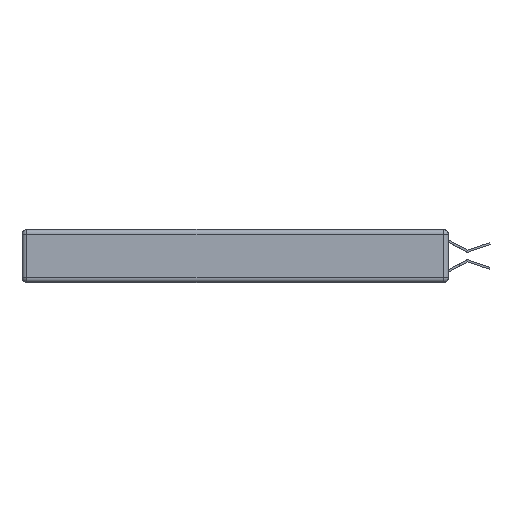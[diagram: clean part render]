
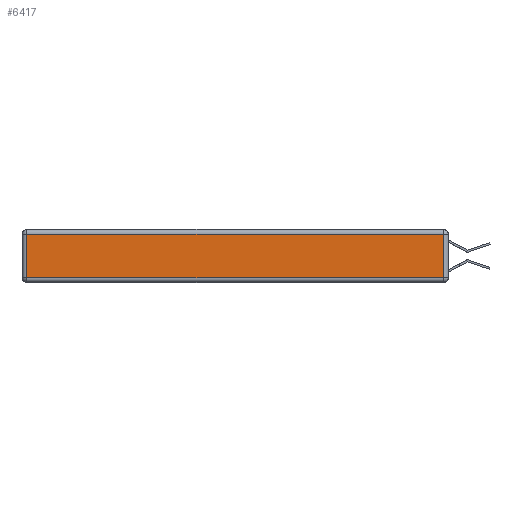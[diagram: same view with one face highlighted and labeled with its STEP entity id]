
A CAD part, left-side view. The second image highlights one B-rep face of the part: STEP entity #6417.
In plain terms, the highlighted planar face has unit normal (-1, 0, 0).
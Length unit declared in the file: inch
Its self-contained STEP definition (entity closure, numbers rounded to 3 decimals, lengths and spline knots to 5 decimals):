
#56 = VERTEX_POINT ( 'NONE', #13258 ) ;
#474 = VECTOR ( 'NONE', #6064, 39.37008 ) ;
#493 = CARTESIAN_POINT ( 'NONE',  ( 0., 2.72, -0.03 ) ) ;
#986 = DIRECTION ( 'NONE',  ( 0., 0., 1. ) ) ;
#1039 = VECTOR ( 'NONE', #4976, 39.37008 ) ;
#2779 = LINE ( 'NONE', #11573, #13890 ) ;
#2848 = LINE ( 'NONE', #9971, #1039 ) ;
#3657 = EDGE_CURVE ( 'NONE', #56, #13476, #2779, .T. ) ;
#4976 = DIRECTION ( 'NONE',  ( 0., 1., 0. ) ) ;
#5623 = EDGE_LOOP ( 'NONE', ( #18469, #15505, #10082, #20493 ) ) ;
#6064 = DIRECTION ( 'NONE',  ( 0., 0., -1. ) ) ;
#6417 = ADVANCED_FACE ( 'NONE', ( #8590 ), #9665, .T. ) ;
#6833 = CARTESIAN_POINT ( 'NONE',  ( 0., 0.03, -0.03 ) ) ;
#7909 = EDGE_CURVE ( 'NONE', #14890, #14992, #2848, .T. ) ;
#8251 = EDGE_CURVE ( 'NONE', #14992, #56, #13700, .T. ) ;
#8590 = FACE_OUTER_BOUND ( 'NONE', #5623, .T. ) ;
#9474 = CARTESIAN_POINT ( 'NONE',  ( 0., 0.03, -0.343 ) ) ;
#9665 = PLANE ( 'NONE',  #17596 ) ;
#9816 = CARTESIAN_POINT ( 'NONE',  ( 0., 0., -0.343 ) ) ;
#9971 = CARTESIAN_POINT ( 'NONE',  ( 0., 2.75, -0.03 ) ) ;
#10082 = ORIENTED_EDGE ( 'NONE', *, *, #7909, .T. ) ;
#10886 = VECTOR ( 'NONE', #986, 39.37008 ) ;
#11407 = DIRECTION ( 'NONE',  ( -1., 0., 0. ) ) ;
#11573 = CARTESIAN_POINT ( 'NONE',  ( 0., 0., -0.313 ) ) ;
#13258 = CARTESIAN_POINT ( 'NONE',  ( 0., 2.72, -0.313 ) ) ;
#13476 = VERTEX_POINT ( 'NONE', #16905 ) ;
#13700 = LINE ( 'NONE', #14168, #474 ) ;
#13890 = VECTOR ( 'NONE', #21432, 39.37008 ) ;
#14020 = EDGE_CURVE ( 'NONE', #13476, #14890, #15289, .T. ) ;
#14168 = CARTESIAN_POINT ( 'NONE',  ( 0., 2.72, -0.343 ) ) ;
#14890 = VERTEX_POINT ( 'NONE', #6833 ) ;
#14992 = VERTEX_POINT ( 'NONE', #493 ) ;
#15289 = LINE ( 'NONE', #9474, #10886 ) ;
#15505 = ORIENTED_EDGE ( 'NONE', *, *, #14020, .T. ) ;
#16475 = DIRECTION ( 'NONE',  ( 0., 0., 1. ) ) ;
#16905 = CARTESIAN_POINT ( 'NONE',  ( 0., 0.03, -0.313 ) ) ;
#17596 = AXIS2_PLACEMENT_3D ( 'NONE', #9816, #11407, #16475 ) ;
#18469 = ORIENTED_EDGE ( 'NONE', *, *, #3657, .T. ) ;
#20493 = ORIENTED_EDGE ( 'NONE', *, *, #8251, .T. ) ;
#21432 = DIRECTION ( 'NONE',  ( 0., -1., 0. ) ) ;
